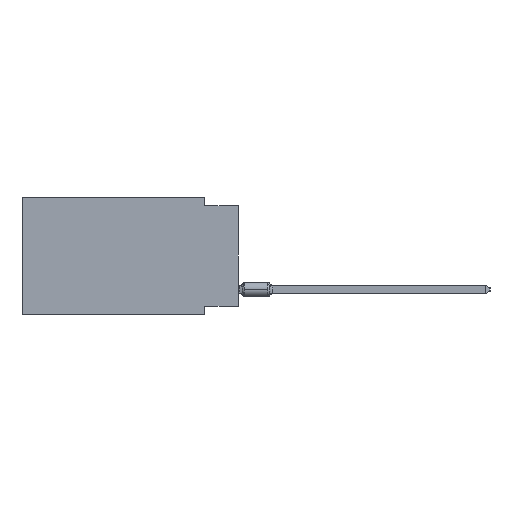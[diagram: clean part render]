
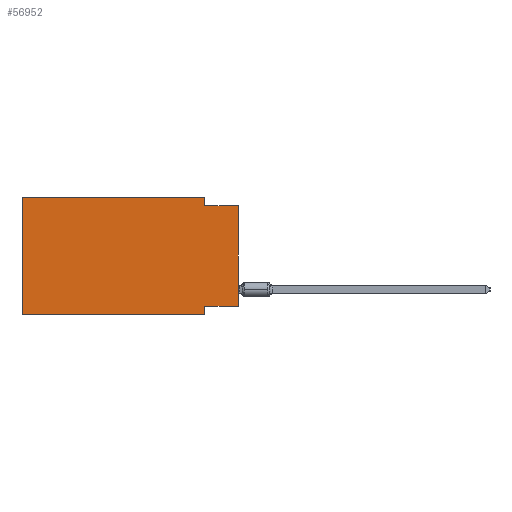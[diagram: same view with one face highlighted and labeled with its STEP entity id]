
A CAD part, left-side view. The second image highlights one B-rep face of the part: STEP entity #56952.
In plain terms, the highlighted planar face has unit normal (-1, 0, 0).
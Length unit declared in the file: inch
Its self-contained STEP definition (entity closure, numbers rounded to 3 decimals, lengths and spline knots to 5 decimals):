
#1436 = DIRECTION ( 'NONE',  ( 0., 0., -1. ) ) ;
#2667 = DIRECTION ( 'NONE',  ( 0., 1., 0. ) ) ;
#5108 = CARTESIAN_POINT ( 'NONE',  ( 0., 0.1, -0.35 ) ) ;
#5719 = VECTOR ( 'NONE', #21473, 39.37008 ) ;
#6296 = CARTESIAN_POINT ( 'NONE',  ( 0., 0.1, -0.35 ) ) ;
#6676 = EDGE_LOOP ( 'NONE', ( #58164, #16012, #17115, #66184, #66756, #27409, #50991, #11872 ) ) ;
#7113 = VECTOR ( 'NONE', #1436, 39.37008 ) ;
#8107 = EDGE_CURVE ( 'NONE', #32855, #41557, #47661, .T. ) ;
#8958 = DIRECTION ( 'NONE',  ( 0., -1., 0. ) ) ;
#9666 = LINE ( 'NONE', #70061, #55786 ) ;
#11733 = EDGE_CURVE ( 'NONE', #17555, #64732, #9666, .T. ) ;
#11872 = ORIENTED_EDGE ( 'NONE', *, *, #8107, .F. ) ;
#14300 = VECTOR ( 'NONE', #43996, 39.37008 ) ;
#14639 = CARTESIAN_POINT ( 'NONE',  ( 0., 0.645, 0. ) ) ;
#16012 = ORIENTED_EDGE ( 'NONE', *, *, #21527, .F. ) ;
#16212 = EDGE_CURVE ( 'NONE', #41557, #62428, #71368, .T. ) ;
#16945 = VECTOR ( 'NONE', #18718, 39.37008 ) ;
#17115 = ORIENTED_EDGE ( 'NONE', *, *, #20159, .F. ) ;
#17555 = VERTEX_POINT ( 'NONE', #14639 ) ;
#18515 = DIRECTION ( 'NONE',  ( 0., -1., 0. ) ) ;
#18718 = DIRECTION ( 'NONE',  ( 0., 0., 1. ) ) ;
#18871 = LINE ( 'NONE', #24707, #63407 ) ;
#19557 = CARTESIAN_POINT ( 'NONE',  ( 0., 0., -0.025 ) ) ;
#20159 = EDGE_CURVE ( 'NONE', #64732, #65272, #68404, .T. ) ;
#21473 = DIRECTION ( 'NONE',  ( 0., 0., -1. ) ) ;
#21527 = EDGE_CURVE ( 'NONE', #65272, #38378, #60844, .T. ) ;
#22643 = CARTESIAN_POINT ( 'NONE',  ( 0., 0.1, 0. ) ) ;
#24707 = CARTESIAN_POINT ( 'NONE',  ( 0., 0.645, -0.35 ) ) ;
#27409 = ORIENTED_EDGE ( 'NONE', *, *, #44029, .T. ) ;
#27872 = CARTESIAN_POINT ( 'NONE',  ( 0., 0., -0.025 ) ) ;
#29351 = CARTESIAN_POINT ( 'NONE',  ( 0., 0., 0. ) ) ;
#29382 = CARTESIAN_POINT ( 'NONE',  ( 0., 0., -0.325 ) ) ;
#31035 = AXIS2_PLACEMENT_3D ( 'NONE', #69843, #58887, #58158 ) ;
#32289 = VECTOR ( 'NONE', #44320, 39.37008 ) ;
#32855 = VERTEX_POINT ( 'NONE', #43544 ) ;
#33495 = VERTEX_POINT ( 'NONE', #63926 ) ;
#37989 = CARTESIAN_POINT ( 'NONE',  ( 0., 0.1, -0.025 ) ) ;
#38378 = VERTEX_POINT ( 'NONE', #19557 ) ;
#41557 = VERTEX_POINT ( 'NONE', #43969 ) ;
#43544 = CARTESIAN_POINT ( 'NONE',  ( 0., 0., -0.325 ) ) ;
#43969 = CARTESIAN_POINT ( 'NONE',  ( 0., 0.1, -0.325 ) ) ;
#43996 = DIRECTION ( 'NONE',  ( 0., -1., 0. ) ) ;
#44029 = EDGE_CURVE ( 'NONE', #33495, #62428, #18871, .T. ) ;
#44320 = DIRECTION ( 'NONE',  ( 0., 0., 1. ) ) ;
#47661 = LINE ( 'NONE', #29382, #59151 ) ;
#48218 = FACE_OUTER_BOUND ( 'NONE', #6676, .T. ) ;
#48634 = EDGE_CURVE ( 'NONE', #32855, #38378, #69245, .T. ) ;
#49820 = CARTESIAN_POINT ( 'NONE',  ( 0., 0.645, 0. ) ) ;
#49991 = EDGE_CURVE ( 'NONE', #33495, #17555, #72144, .T. ) ;
#50991 = ORIENTED_EDGE ( 'NONE', *, *, #16212, .F. ) ;
#55786 = VECTOR ( 'NONE', #8958, 39.37008 ) ;
#56952 = ADVANCED_FACE ( 'NONE', ( #48218 ), #69486, .F. ) ;
#58158 = DIRECTION ( 'NONE',  ( 0., 0., -1. ) ) ;
#58164 = ORIENTED_EDGE ( 'NONE', *, *, #48634, .T. ) ;
#58887 = DIRECTION ( 'NONE',  ( 1., 0., 0. ) ) ;
#59151 = VECTOR ( 'NONE', #2667, 39.37008 ) ;
#60844 = LINE ( 'NONE', #27872, #14300 ) ;
#62428 = VERTEX_POINT ( 'NONE', #6296 ) ;
#62762 = CARTESIAN_POINT ( 'NONE',  ( 0., 0.1, 0. ) ) ;
#63407 = VECTOR ( 'NONE', #18515, 39.37008 ) ;
#63926 = CARTESIAN_POINT ( 'NONE',  ( 0., 0.645, -0.35 ) ) ;
#64732 = VERTEX_POINT ( 'NONE', #62762 ) ;
#65272 = VERTEX_POINT ( 'NONE', #37989 ) ;
#66184 = ORIENTED_EDGE ( 'NONE', *, *, #11733, .F. ) ;
#66756 = ORIENTED_EDGE ( 'NONE', *, *, #49991, .F. ) ;
#68404 = LINE ( 'NONE', #22643, #7113 ) ;
#69245 = LINE ( 'NONE', #29351, #16945 ) ;
#69486 = PLANE ( 'NONE',  #31035 ) ;
#69843 = CARTESIAN_POINT ( 'NONE',  ( 0., 0.645, 0. ) ) ;
#70061 = CARTESIAN_POINT ( 'NONE',  ( 0., 0.645, 0. ) ) ;
#71368 = LINE ( 'NONE', #5108, #5719 ) ;
#72144 = LINE ( 'NONE', #49820, #32289 ) ;
